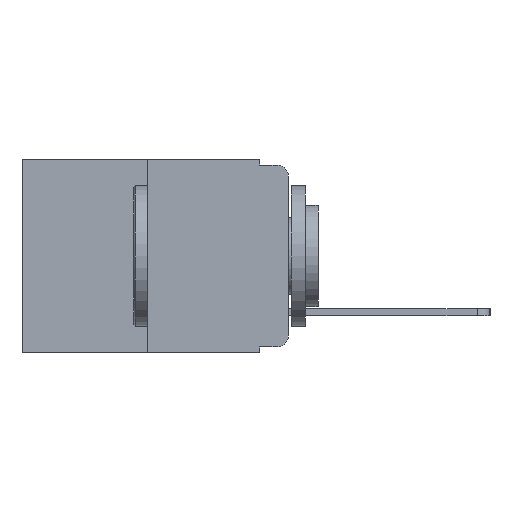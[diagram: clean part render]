
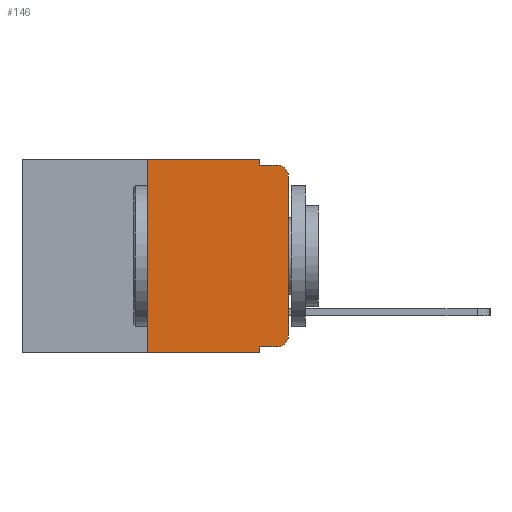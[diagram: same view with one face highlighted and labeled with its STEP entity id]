
A CAD part, left-side view. The second image highlights one B-rep face of the part: STEP entity #146.
In plain terms, the highlighted planar face has unit normal (-1, 0, 0).
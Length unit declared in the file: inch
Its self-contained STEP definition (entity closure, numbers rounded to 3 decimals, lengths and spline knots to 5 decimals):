
#51 = LINE ( 'NONE', #7603, #3205 ) ;
#130 = CARTESIAN_POINT ( 'NONE',  ( 0., 0.473, 0. ) ) ;
#146 = ADVANCED_FACE ( 'NONE', ( #14738 ), #15639, .F. ) ;
#180 = VECTOR ( 'NONE', #15609, 39.37008 ) ;
#330 = ORIENTED_EDGE ( 'NONE', *, *, #5274, .F. ) ;
#489 = ORIENTED_EDGE ( 'NONE', *, *, #7917, .F. ) ;
#627 = ORIENTED_EDGE ( 'NONE', *, *, #8641, .T. ) ;
#1510 = VERTEX_POINT ( 'NONE', #10042 ) ;
#1899 = ORIENTED_EDGE ( 'NONE', *, *, #10366, .T. ) ;
#2327 = CARTESIAN_POINT ( 'NONE',  ( 0., 0.02, -0.333 ) ) ;
#2390 = LINE ( 'NONE', #5889, #14941 ) ;
#2553 = ORIENTED_EDGE ( 'NONE', *, *, #10269, .F. ) ;
#2661 = ORIENTED_EDGE ( 'NONE', *, *, #4080, .T. ) ;
#2768 = DIRECTION ( 'NONE',  ( 0., -1., 0. ) ) ;
#2789 = VERTEX_POINT ( 'NONE', #4005 ) ;
#2914 = EDGE_CURVE ( 'NONE', #9444, #6954, #9416, .T. ) ;
#3019 = CARTESIAN_POINT ( 'NONE',  ( 0., 0.051, 0. ) ) ;
#3205 = VECTOR ( 'NONE', #16199, 39.37008 ) ;
#3360 = CARTESIAN_POINT ( 'NONE',  ( 0., 0., 0. ) ) ;
#3394 = CIRCLE ( 'NONE', #8802, 0.02 ) ;
#3443 = CARTESIAN_POINT ( 'NONE',  ( 0., 0.02, -0.01 ) ) ;
#3602 = LINE ( 'NONE', #130, #15641 ) ;
#4005 = CARTESIAN_POINT ( 'NONE',  ( 0., 0.051, -0.333 ) ) ;
#4080 = EDGE_CURVE ( 'NONE', #2789, #5037, #7205, .T. ) ;
#4205 = VECTOR ( 'NONE', #2768, 39.37008 ) ;
#4234 = CARTESIAN_POINT ( 'NONE',  ( 0., 0.02, -0.03 ) ) ;
#4242 = VECTOR ( 'NONE', #10788, 39.37008 ) ;
#4422 = CARTESIAN_POINT ( 'NONE',  ( 0., 0.051, -0.343 ) ) ;
#4501 = DIRECTION ( 'NONE',  ( 1., 0., 0. ) ) ;
#4637 = CARTESIAN_POINT ( 'NONE',  ( 0., 0.051, -0.01 ) ) ;
#4652 = DIRECTION ( 'NONE',  ( 0., 0., 1. ) ) ;
#4713 = DIRECTION ( 'NONE',  ( -1., 0., 0. ) ) ;
#4795 = EDGE_LOOP ( 'NONE', ( #5192, #6163, #7177, #7428, #330, #489, #1899, #2553, #2661, #627 ) ) ;
#4873 = VERTEX_POINT ( 'NONE', #9685 ) ;
#4880 = EDGE_CURVE ( 'NONE', #6954, #8171, #2390, .T. ) ;
#5037 = VERTEX_POINT ( 'NONE', #2327 ) ;
#5192 = ORIENTED_EDGE ( 'NONE', *, *, #6677, .T. ) ;
#5274 = EDGE_CURVE ( 'NONE', #4873, #9444, #3602, .T. ) ;
#5471 = DIRECTION ( 'NONE',  ( 0., 0., -1. ) ) ;
#5531 = VECTOR ( 'NONE', #4652, 39.37008 ) ;
#5636 = VECTOR ( 'NONE', #11891, 39.37008 ) ;
#5889 = CARTESIAN_POINT ( 'NONE',  ( 0., 0.051, -0.01 ) ) ;
#5926 = LINE ( 'NONE', #3360, #5531 ) ;
#6163 = ORIENTED_EDGE ( 'NONE', *, *, #10442, .T. ) ;
#6677 = EDGE_CURVE ( 'NONE', #1510, #11818, #5926, .T. ) ;
#6682 = LINE ( 'NONE', #12005, #180 ) ;
#6954 = VERTEX_POINT ( 'NONE', #4637 ) ;
#7177 = ORIENTED_EDGE ( 'NONE', *, *, #4880, .F. ) ;
#7205 = LINE ( 'NONE', #9485, #4242 ) ;
#7428 = ORIENTED_EDGE ( 'NONE', *, *, #2914, .F. ) ;
#7603 = CARTESIAN_POINT ( 'NONE',  ( 0., 0.051, 0. ) ) ;
#7917 = EDGE_CURVE ( 'NONE', #11828, #4873, #6682, .T. ) ;
#8171 = VERTEX_POINT ( 'NONE', #3443 ) ;
#8330 = AXIS2_PLACEMENT_3D ( 'NONE', #12269, #4713, #13483 ) ;
#8641 = EDGE_CURVE ( 'NONE', #5037, #1510, #15146, .T. ) ;
#8802 = AXIS2_PLACEMENT_3D ( 'NONE', #4234, #13025, #5471 ) ;
#9416 = LINE ( 'NONE', #3019, #5636 ) ;
#9444 = VERTEX_POINT ( 'NONE', #10307 ) ;
#9485 = CARTESIAN_POINT ( 'NONE',  ( 0., 0.051, -0.333 ) ) ;
#9685 = CARTESIAN_POINT ( 'NONE',  ( 0., 0.25, 0. ) ) ;
#9741 = DIRECTION ( 'NONE',  ( 0., -1., 0. ) ) ;
#10042 = CARTESIAN_POINT ( 'NONE',  ( 0., 0., -0.313 ) ) ;
#10142 = CARTESIAN_POINT ( 'NONE',  ( 0., 0.25, -0.343 ) ) ;
#10269 = EDGE_CURVE ( 'NONE', #2789, #11444, #51, .T. ) ;
#10307 = CARTESIAN_POINT ( 'NONE',  ( 0., 0.051, 0. ) ) ;
#10366 = EDGE_CURVE ( 'NONE', #11828, #11444, #14174, .T. ) ;
#10442 = EDGE_CURVE ( 'NONE', #11818, #8171, #3394, .T. ) ;
#10484 = DIRECTION ( 'NONE',  ( 0., -1., 0. ) ) ;
#10788 = DIRECTION ( 'NONE',  ( 0., -1., 0. ) ) ;
#11412 = CARTESIAN_POINT ( 'NONE',  ( 0., 0., -0.03 ) ) ;
#11423 = AXIS2_PLACEMENT_3D ( 'NONE', #13946, #4501, #12007 ) ;
#11444 = VERTEX_POINT ( 'NONE', #4422 ) ;
#11818 = VERTEX_POINT ( 'NONE', #11412 ) ;
#11828 = VERTEX_POINT ( 'NONE', #10142 ) ;
#11891 = DIRECTION ( 'NONE',  ( 0., 0., -1. ) ) ;
#12005 = CARTESIAN_POINT ( 'NONE',  ( 0., 0.25, 0. ) ) ;
#12007 = DIRECTION ( 'NONE',  ( 0., 0., -1. ) ) ;
#12269 = CARTESIAN_POINT ( 'NONE',  ( 0., 0.02, -0.313 ) ) ;
#12826 = CARTESIAN_POINT ( 'NONE',  ( 0., 0.473, -0.343 ) ) ;
#13025 = DIRECTION ( 'NONE',  ( -1., 0., 0. ) ) ;
#13483 = DIRECTION ( 'NONE',  ( 0., 0., -1. ) ) ;
#13946 = CARTESIAN_POINT ( 'NONE',  ( 0., 0.473, 0. ) ) ;
#14174 = LINE ( 'NONE', #12826, #4205 ) ;
#14738 = FACE_OUTER_BOUND ( 'NONE', #4795, .T. ) ;
#14941 = VECTOR ( 'NONE', #9741, 39.37008 ) ;
#15146 = CIRCLE ( 'NONE', #8330, 0.02 ) ;
#15609 = DIRECTION ( 'NONE',  ( 0., 0., 1. ) ) ;
#15639 = PLANE ( 'NONE',  #11423 ) ;
#15641 = VECTOR ( 'NONE', #10484, 39.37008 ) ;
#16199 = DIRECTION ( 'NONE',  ( 0., 0., -1. ) ) ;
